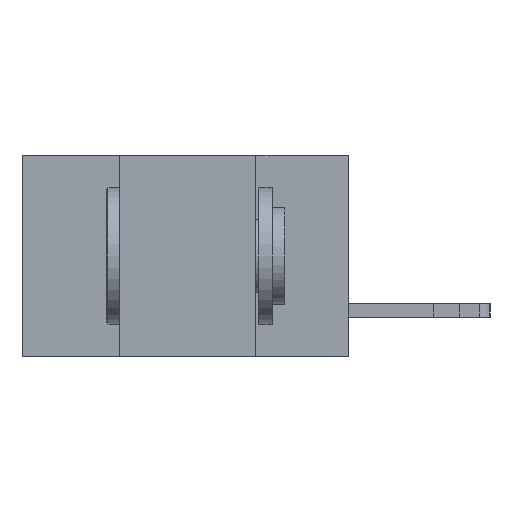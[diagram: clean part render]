
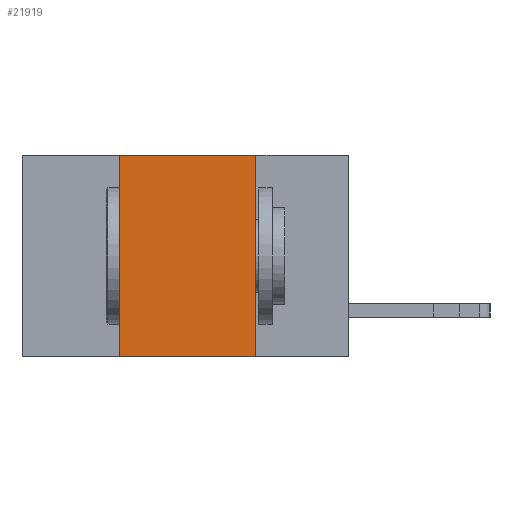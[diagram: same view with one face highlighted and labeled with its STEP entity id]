
A CAD part, left-side view. The second image highlights one B-rep face of the part: STEP entity #21919.
In plain terms, the highlighted planar face has unit normal (-1, 0, 0).
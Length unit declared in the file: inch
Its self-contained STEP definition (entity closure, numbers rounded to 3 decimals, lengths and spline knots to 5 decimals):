
#33 = EDGE_CURVE ( 'NONE', #10424, #16399, #1962, .T. ) ;
#773 = ORIENTED_EDGE ( 'NONE', *, *, #16245, .F. ) ;
#1398 = EDGE_LOOP ( 'NONE', ( #8800, #773, #16306, #5430 ) ) ;
#1595 = DIRECTION ( 'NONE',  ( 1., 0., 0. ) ) ;
#1962 = LINE ( 'NONE', #2941, #19635 ) ;
#2840 = DIRECTION ( 'NONE',  ( 0., 0., 1. ) ) ;
#2941 = CARTESIAN_POINT ( 'NONE',  ( 0., 0.42, 0. ) ) ;
#2979 = VERTEX_POINT ( 'NONE', #8107 ) ;
#4348 = LINE ( 'NONE', #21579, #4908 ) ;
#4908 = VECTOR ( 'NONE', #16463, 39.37008 ) ;
#5067 = AXIS2_PLACEMENT_3D ( 'NONE', #12311, #1595, #14099 ) ;
#5430 = ORIENTED_EDGE ( 'NONE', *, *, #9877, .T. ) ;
#7398 = LINE ( 'NONE', #11766, #11603 ) ;
#8107 = CARTESIAN_POINT ( 'NONE',  ( 0., 0.17, 0. ) ) ;
#8800 = ORIENTED_EDGE ( 'NONE', *, *, #12916, .F. ) ;
#9877 = EDGE_CURVE ( 'NONE', #10424, #16327, #7398, .T. ) ;
#10044 = CARTESIAN_POINT ( 'NONE',  ( 0., 0.17, -0.37 ) ) ;
#10424 = VERTEX_POINT ( 'NONE', #21954 ) ;
#11453 = LINE ( 'NONE', #20195, #16138 ) ;
#11603 = VECTOR ( 'NONE', #20438, 39.37008 ) ;
#11766 = CARTESIAN_POINT ( 'NONE',  ( 0., 0.6, -0.37 ) ) ;
#12311 = CARTESIAN_POINT ( 'NONE',  ( 0., 0.6, 0. ) ) ;
#12916 = EDGE_CURVE ( 'NONE', #2979, #16327, #4348, .T. ) ;
#14099 = DIRECTION ( 'NONE',  ( 0., 0., -1. ) ) ;
#15463 = CARTESIAN_POINT ( 'NONE',  ( 0., 0.42, 0. ) ) ;
#16138 = VECTOR ( 'NONE', #21899, 39.37008 ) ;
#16245 = EDGE_CURVE ( 'NONE', #16399, #2979, #11453, .T. ) ;
#16306 = ORIENTED_EDGE ( 'NONE', *, *, #33, .F. ) ;
#16327 = VERTEX_POINT ( 'NONE', #10044 ) ;
#16399 = VERTEX_POINT ( 'NONE', #15463 ) ;
#16463 = DIRECTION ( 'NONE',  ( 0., 0., -1. ) ) ;
#18018 = FACE_OUTER_BOUND ( 'NONE', #1398, .T. ) ;
#19635 = VECTOR ( 'NONE', #2840, 39.37008 ) ;
#20195 = CARTESIAN_POINT ( 'NONE',  ( 0., 0.6, 0. ) ) ;
#20438 = DIRECTION ( 'NONE',  ( 0., -1., 0. ) ) ;
#21579 = CARTESIAN_POINT ( 'NONE',  ( 0., 0.17, 0. ) ) ;
#21899 = DIRECTION ( 'NONE',  ( 0., -1., 0. ) ) ;
#21919 = ADVANCED_FACE ( 'NONE', ( #18018 ), #22595, .F. ) ;
#21954 = CARTESIAN_POINT ( 'NONE',  ( 0., 0.42, -0.37 ) ) ;
#22595 = PLANE ( 'NONE',  #5067 ) ;
